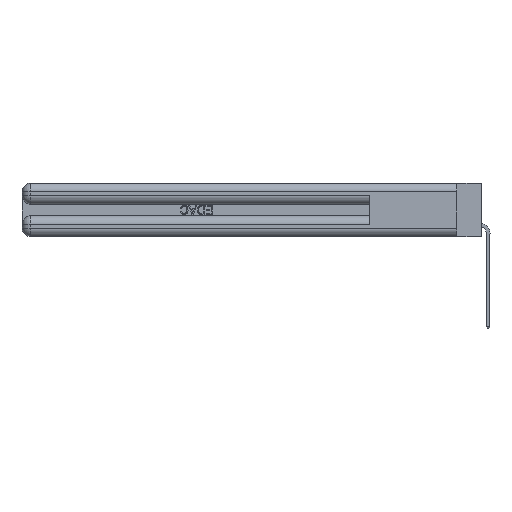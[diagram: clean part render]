
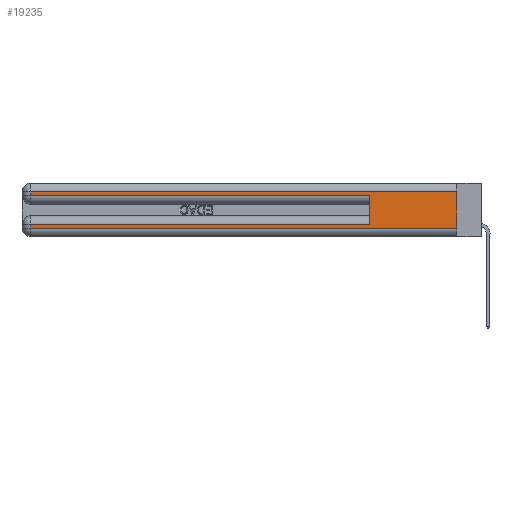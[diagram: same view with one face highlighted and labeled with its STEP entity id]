
A CAD part, left-side view. The second image highlights one B-rep face of the part: STEP entity #19235.
In plain terms, the highlighted planar face has unit normal (-1, 0, 0).
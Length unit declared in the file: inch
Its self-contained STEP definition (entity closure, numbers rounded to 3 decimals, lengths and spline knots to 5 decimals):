
#10 = VECTOR ( 'NONE', #29658, 39.37008 ) ;
#1065 = VECTOR ( 'NONE', #6103, 39.37008 ) ;
#2674 = LINE ( 'NONE', #40633, #5609 ) ;
#4449 = LINE ( 'NONE', #20236, #10842 ) ;
#5464 = ORIENTED_EDGE ( 'NONE', *, *, #22997, .T. ) ;
#5609 = VECTOR ( 'NONE', #34728, 39.37008 ) ;
#6103 = DIRECTION ( 'NONE',  ( 0., 1., 0. ) ) ;
#7498 = VERTEX_POINT ( 'NONE', #31232 ) ;
#7622 = CARTESIAN_POINT ( 'NONE',  ( 0., 2.94, 0.37 ) ) ;
#8616 = VERTEX_POINT ( 'NONE', #34184 ) ;
#9850 = LINE ( 'NONE', #31557, #1065 ) ;
#10100 = ORIENTED_EDGE ( 'NONE', *, *, #34414, .T. ) ;
#10842 = VECTOR ( 'NONE', #32793, 39.37008 ) ;
#11362 = PLANE ( 'NONE',  #23117 ) ;
#11474 = CARTESIAN_POINT ( 'NONE',  ( 0., 0., 0.31 ) ) ;
#11578 = DIRECTION ( 'NONE',  ( 0., 0., -1. ) ) ;
#12266 = LINE ( 'NONE', #7622, #10 ) ;
#12403 = ORIENTED_EDGE ( 'NONE', *, *, #22940, .T. ) ;
#12681 = EDGE_LOOP ( 'NONE', ( #26653, #12403, #36603, #5464, #38936, #39498, #10100, #22228 ) ) ;
#12721 = FACE_OUTER_BOUND ( 'NONE', #12681, .T. ) ;
#12740 = VECTOR ( 'NONE', #15987, 39.37008 ) ;
#12751 = VERTEX_POINT ( 'NONE', #38674 ) ;
#13100 = VERTEX_POINT ( 'NONE', #11474 ) ;
#14645 = DIRECTION ( 'NONE',  ( 0., 0., -1. ) ) ;
#15987 = DIRECTION ( 'NONE',  ( 0., 0., 1. ) ) ;
#17436 = EDGE_CURVE ( 'NONE', #33916, #22573, #22763, .T. ) ;
#17808 = VECTOR ( 'NONE', #23665, 39.37008 ) ;
#18734 = CARTESIAN_POINT ( 'NONE',  ( 0., 0., 0.06 ) ) ;
#19235 = ADVANCED_FACE ( 'NONE', ( #12721 ), #11362, .F. ) ;
#20236 = CARTESIAN_POINT ( 'NONE',  ( 0., 0., 0.31 ) ) ;
#20340 = LINE ( 'NONE', #18734, #35634 ) ;
#20477 = CARTESIAN_POINT ( 'NONE',  ( 0., 0., 0.06 ) ) ;
#21532 = DIRECTION ( 'NONE',  ( 1., 0., 0. ) ) ;
#22118 = DIRECTION ( 'NONE',  ( 0., -1., 0. ) ) ;
#22228 = ORIENTED_EDGE ( 'NONE', *, *, #30669, .T. ) ;
#22573 = VERTEX_POINT ( 'NONE', #33929 ) ;
#22763 = LINE ( 'NONE', #33225, #35601 ) ;
#22940 = EDGE_CURVE ( 'NONE', #13100, #33916, #4449, .T. ) ;
#22997 = EDGE_CURVE ( 'NONE', #22573, #8616, #34977, .T. ) ;
#23117 = AXIS2_PLACEMENT_3D ( 'NONE', #33548, #21532, #14645 ) ;
#23665 = DIRECTION ( 'NONE',  ( 0., -1., 0. ) ) ;
#23975 = EDGE_CURVE ( 'NONE', #7498, #8616, #25572, .T. ) ;
#25572 = LINE ( 'NONE', #37906, #12740 ) ;
#26653 = ORIENTED_EDGE ( 'NONE', *, *, #27230, .F. ) ;
#27230 = EDGE_CURVE ( 'NONE', #13100, #37145, #2674, .T. ) ;
#29658 = DIRECTION ( 'NONE',  ( 0., 0., -1. ) ) ;
#30669 = EDGE_CURVE ( 'NONE', #35911, #37145, #20340, .T. ) ;
#31232 = CARTESIAN_POINT ( 'NONE',  ( 0., 0.6, 0.085 ) ) ;
#31557 = CARTESIAN_POINT ( 'NONE',  ( 0., 0., 0.085 ) ) ;
#31966 = CARTESIAN_POINT ( 'NONE',  ( 0., 2.94, 0.06 ) ) ;
#32077 = EDGE_CURVE ( 'NONE', #7498, #12751, #9850, .T. ) ;
#32793 = DIRECTION ( 'NONE',  ( 0., 1., 0. ) ) ;
#33225 = CARTESIAN_POINT ( 'NONE',  ( 0., 2.94, 0.37 ) ) ;
#33548 = CARTESIAN_POINT ( 'NONE',  ( 0., 0., 0.37 ) ) ;
#33916 = VERTEX_POINT ( 'NONE', #36949 ) ;
#33929 = CARTESIAN_POINT ( 'NONE',  ( 0., 2.94, 0.285 ) ) ;
#34184 = CARTESIAN_POINT ( 'NONE',  ( 0., 0.6, 0.285 ) ) ;
#34414 = EDGE_CURVE ( 'NONE', #12751, #35911, #12266, .T. ) ;
#34728 = DIRECTION ( 'NONE',  ( 0., 0., -1. ) ) ;
#34977 = LINE ( 'NONE', #39083, #17808 ) ;
#35601 = VECTOR ( 'NONE', #11578, 39.37008 ) ;
#35634 = VECTOR ( 'NONE', #22118, 39.37008 ) ;
#35911 = VERTEX_POINT ( 'NONE', #31966 ) ;
#36603 = ORIENTED_EDGE ( 'NONE', *, *, #17436, .T. ) ;
#36949 = CARTESIAN_POINT ( 'NONE',  ( 0., 2.94, 0.31 ) ) ;
#37145 = VERTEX_POINT ( 'NONE', #20477 ) ;
#37906 = CARTESIAN_POINT ( 'NONE',  ( 0., 0.6, 0.145 ) ) ;
#38674 = CARTESIAN_POINT ( 'NONE',  ( 0., 2.94, 0.085 ) ) ;
#38936 = ORIENTED_EDGE ( 'NONE', *, *, #23975, .F. ) ;
#39083 = CARTESIAN_POINT ( 'NONE',  ( 0., 0., 0.285 ) ) ;
#39498 = ORIENTED_EDGE ( 'NONE', *, *, #32077, .T. ) ;
#40633 = CARTESIAN_POINT ( 'NONE',  ( 0., 0., 0.37 ) ) ;
